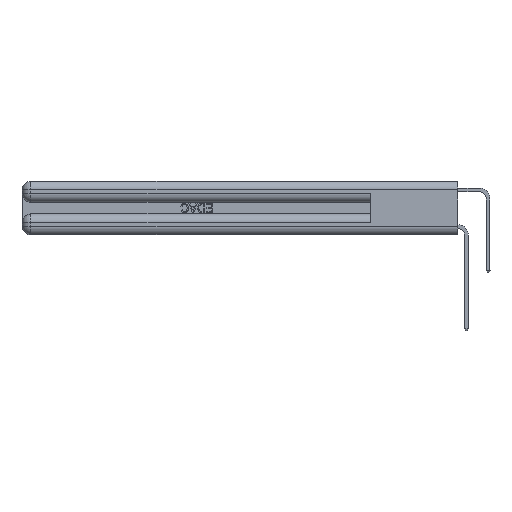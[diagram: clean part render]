
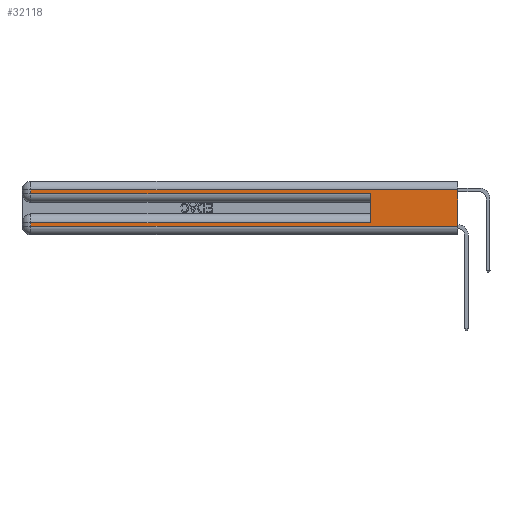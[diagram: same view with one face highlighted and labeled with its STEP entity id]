
A CAD part, left-side view. The second image highlights one B-rep face of the part: STEP entity #32118.
In plain terms, the highlighted planar face has unit normal (-1, 0, 0).
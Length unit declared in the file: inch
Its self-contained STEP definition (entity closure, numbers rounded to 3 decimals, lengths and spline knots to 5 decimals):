
#929 = VECTOR ( 'NONE', #12407, 39.37008 ) ;
#960 = VECTOR ( 'NONE', #34716, 39.37008 ) ;
#1028 = VERTEX_POINT ( 'NONE', #25800 ) ;
#1245 = VERTEX_POINT ( 'NONE', #14905 ) ;
#1246 = CARTESIAN_POINT ( 'NONE',  ( 0., 2.94, 0.37 ) ) ;
#1935 = CARTESIAN_POINT ( 'NONE',  ( 0., 0., 0.085 ) ) ;
#3126 = CARTESIAN_POINT ( 'NONE',  ( 0., 0., 0.37 ) ) ;
#3285 = VECTOR ( 'NONE', #9828, 39.37008 ) ;
#3888 = DIRECTION ( 'NONE',  ( 1., 0., 0. ) ) ;
#3987 = LINE ( 'NONE', #36493, #3285 ) ;
#4666 = VECTOR ( 'NONE', #35726, 39.37008 ) ;
#4786 = ORIENTED_EDGE ( 'NONE', *, *, #29914, .T. ) ;
#5179 = ORIENTED_EDGE ( 'NONE', *, *, #31075, .F. ) ;
#5381 = CARTESIAN_POINT ( 'NONE',  ( 0., 0., 0.31 ) ) ;
#6948 = LINE ( 'NONE', #7139, #929 ) ;
#7139 = CARTESIAN_POINT ( 'NONE',  ( 0., 0., 0.06 ) ) ;
#7517 = EDGE_LOOP ( 'NONE', ( #19878, #26747, #13706, #32589, #5179, #37311, #4786, #14542 ) ) ;
#8370 = VECTOR ( 'NONE', #38016, 39.37008 ) ;
#9693 = VERTEX_POINT ( 'NONE', #30607 ) ;
#9828 = DIRECTION ( 'NONE',  ( 0., 0., -1. ) ) ;
#10348 = CARTESIAN_POINT ( 'NONE',  ( 0., 0., 0.06 ) ) ;
#11583 = LINE ( 'NONE', #23251, #26354 ) ;
#12207 = VERTEX_POINT ( 'NONE', #35584 ) ;
#12407 = DIRECTION ( 'NONE',  ( 0., -1., 0. ) ) ;
#13706 = ORIENTED_EDGE ( 'NONE', *, *, #17204, .T. ) ;
#14281 = LINE ( 'NONE', #25745, #8370 ) ;
#14542 = ORIENTED_EDGE ( 'NONE', *, *, #29338, .T. ) ;
#14905 = CARTESIAN_POINT ( 'NONE',  ( 0., 2.94, 0.285 ) ) ;
#15916 = AXIS2_PLACEMENT_3D ( 'NONE', #3126, #3888, #24316 ) ;
#16229 = VERTEX_POINT ( 'NONE', #26328 ) ;
#17204 = EDGE_CURVE ( 'NONE', #9693, #1245, #3987, .T. ) ;
#18235 = VERTEX_POINT ( 'NONE', #18892 ) ;
#18892 = CARTESIAN_POINT ( 'NONE',  ( 0., 0.6, 0.085 ) ) ;
#19344 = VERTEX_POINT ( 'NONE', #24336 ) ;
#19878 = ORIENTED_EDGE ( 'NONE', *, *, #28783, .F. ) ;
#20346 = DIRECTION ( 'NONE',  ( 0., -1., 0. ) ) ;
#22973 = VERTEX_POINT ( 'NONE', #10348 ) ;
#23251 = CARTESIAN_POINT ( 'NONE',  ( 0., 0., 0.285 ) ) ;
#24316 = DIRECTION ( 'NONE',  ( 0., 0., -1. ) ) ;
#24336 = CARTESIAN_POINT ( 'NONE',  ( 0., 2.94, 0.06 ) ) ;
#25668 = DIRECTION ( 'NONE',  ( 0., 1., 0. ) ) ;
#25745 = CARTESIAN_POINT ( 'NONE',  ( 0., 0., 0.37 ) ) ;
#25800 = CARTESIAN_POINT ( 'NONE',  ( 0., 2.94, 0.085 ) ) ;
#26195 = DIRECTION ( 'NONE',  ( 0., 1., 0. ) ) ;
#26328 = CARTESIAN_POINT ( 'NONE',  ( 0., 0.6, 0.285 ) ) ;
#26354 = VECTOR ( 'NONE', #20346, 39.37008 ) ;
#26368 = LINE ( 'NONE', #32424, #4666 ) ;
#26449 = EDGE_CURVE ( 'NONE', #12207, #9693, #32055, .T. ) ;
#26747 = ORIENTED_EDGE ( 'NONE', *, *, #26449, .T. ) ;
#26854 = PLANE ( 'NONE',  #15916 ) ;
#28383 = EDGE_CURVE ( 'NONE', #1245, #16229, #11583, .T. ) ;
#28598 = LINE ( 'NONE', #1935, #36209 ) ;
#28680 = LINE ( 'NONE', #1246, #960 ) ;
#28783 = EDGE_CURVE ( 'NONE', #12207, #22973, #14281, .T. ) ;
#29338 = EDGE_CURVE ( 'NONE', #19344, #22973, #6948, .T. ) ;
#29914 = EDGE_CURVE ( 'NONE', #1028, #19344, #28680, .T. ) ;
#30607 = CARTESIAN_POINT ( 'NONE',  ( 0., 2.94, 0.31 ) ) ;
#31075 = EDGE_CURVE ( 'NONE', #18235, #16229, #26368, .T. ) ;
#32055 = LINE ( 'NONE', #5381, #36846 ) ;
#32118 = ADVANCED_FACE ( 'NONE', ( #33473 ), #26854, .F. ) ;
#32424 = CARTESIAN_POINT ( 'NONE',  ( 0., 0.6, 0.145 ) ) ;
#32589 = ORIENTED_EDGE ( 'NONE', *, *, #28383, .T. ) ;
#33473 = FACE_OUTER_BOUND ( 'NONE', #7517, .T. ) ;
#34716 = DIRECTION ( 'NONE',  ( 0., 0., -1. ) ) ;
#35584 = CARTESIAN_POINT ( 'NONE',  ( 0., 0., 0.31 ) ) ;
#35726 = DIRECTION ( 'NONE',  ( 0., 0., 1. ) ) ;
#36209 = VECTOR ( 'NONE', #25668, 39.37008 ) ;
#36493 = CARTESIAN_POINT ( 'NONE',  ( 0., 2.94, 0.37 ) ) ;
#36846 = VECTOR ( 'NONE', #26195, 39.37008 ) ;
#37311 = ORIENTED_EDGE ( 'NONE', *, *, #37925, .T. ) ;
#37925 = EDGE_CURVE ( 'NONE', #18235, #1028, #28598, .T. ) ;
#38016 = DIRECTION ( 'NONE',  ( 0., 0., -1. ) ) ;
